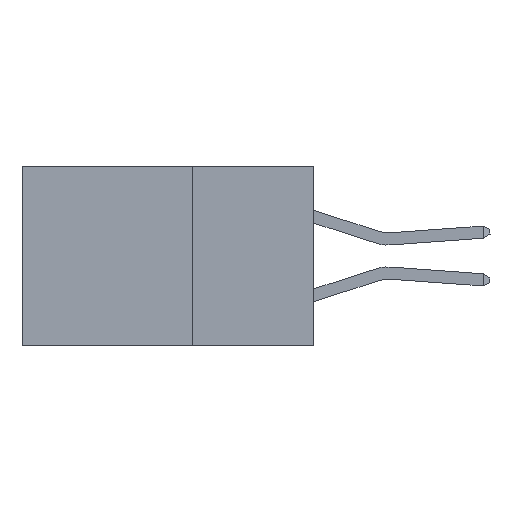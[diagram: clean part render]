
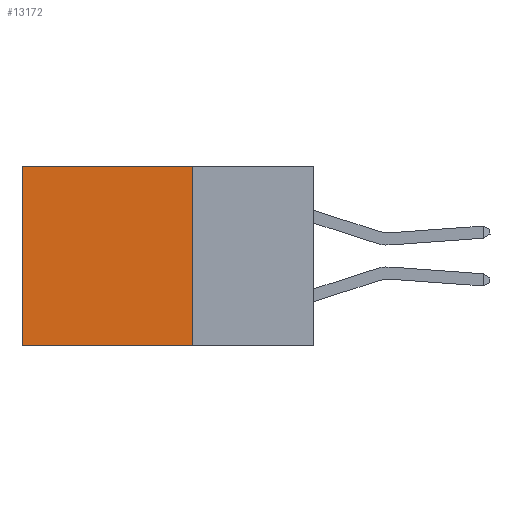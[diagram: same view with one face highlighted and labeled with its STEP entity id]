
A CAD part, left-side view. The second image highlights one B-rep face of the part: STEP entity #13172.
In plain terms, the highlighted planar face has unit normal (-1, 0, 0).
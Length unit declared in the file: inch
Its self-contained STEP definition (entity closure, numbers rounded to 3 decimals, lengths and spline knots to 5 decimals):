
#22 = ORIENTED_EDGE ( 'NONE', *, *, #11337, .F. ) ;
#106 = VECTOR ( 'NONE', #19397, 39.37008 ) ;
#858 = CARTESIAN_POINT ( 'NONE',  ( 0.2875, 0.6, 0. ) ) ;
#1462 = VERTEX_POINT ( 'NONE', #20806 ) ;
#1597 = CARTESIAN_POINT ( 'NONE',  ( 0.2875, 0.25, 0. ) ) ;
#2873 = DIRECTION ( 'NONE',  ( 1., 0., 0. ) ) ;
#3377 = VERTEX_POINT ( 'NONE', #4167 ) ;
#4167 = CARTESIAN_POINT ( 'NONE',  ( 0.2875, 0.25, -0.37 ) ) ;
#4587 = LINE ( 'NONE', #20984, #106 ) ;
#5006 = CARTESIAN_POINT ( 'NONE',  ( 0.2875, 0.6, 0. ) ) ;
#5572 = LINE ( 'NONE', #5006, #8965 ) ;
#5601 = VERTEX_POINT ( 'NONE', #1597 ) ;
#6746 = EDGE_LOOP ( 'NONE', ( #21230, #22, #9424, #15905 ) ) ;
#7415 = CARTESIAN_POINT ( 'NONE',  ( 0.2875, 0.25, 0. ) ) ;
#8239 = CARTESIAN_POINT ( 'NONE',  ( 0.2875, 0.25, -0.37 ) ) ;
#8553 = EDGE_CURVE ( 'NONE', #9463, #1462, #5572, .T. ) ;
#8965 = VECTOR ( 'NONE', #14966, 39.37008 ) ;
#9424 = ORIENTED_EDGE ( 'NONE', *, *, #13683, .F. ) ;
#9463 = VERTEX_POINT ( 'NONE', #858 ) ;
#9910 = DIRECTION ( 'NONE',  ( 0., 1., 0. ) ) ;
#11337 = EDGE_CURVE ( 'NONE', #3377, #1462, #11668, .T. ) ;
#11668 = LINE ( 'NONE', #8239, #19756 ) ;
#12855 = VECTOR ( 'NONE', #15663, 39.37008 ) ;
#13172 = ADVANCED_FACE ( 'NONE', ( #19677 ), #17585, .F. ) ;
#13237 = EDGE_CURVE ( 'NONE', #5601, #9463, #4587, .T. ) ;
#13683 = EDGE_CURVE ( 'NONE', #5601, #3377, #17156, .T. ) ;
#14401 = DIRECTION ( 'NONE',  ( 0., 0., -1. ) ) ;
#14485 = AXIS2_PLACEMENT_3D ( 'NONE', #17520, #2873, #14401 ) ;
#14966 = DIRECTION ( 'NONE',  ( 0., 0., -1. ) ) ;
#15663 = DIRECTION ( 'NONE',  ( 0., 0., -1. ) ) ;
#15905 = ORIENTED_EDGE ( 'NONE', *, *, #13237, .T. ) ;
#17156 = LINE ( 'NONE', #7415, #12855 ) ;
#17520 = CARTESIAN_POINT ( 'NONE',  ( 0.2875, 0.25, 0. ) ) ;
#17585 = PLANE ( 'NONE',  #14485 ) ;
#19397 = DIRECTION ( 'NONE',  ( 0., 1., 0. ) ) ;
#19677 = FACE_OUTER_BOUND ( 'NONE', #6746, .T. ) ;
#19756 = VECTOR ( 'NONE', #9910, 39.37008 ) ;
#20806 = CARTESIAN_POINT ( 'NONE',  ( 0.2875, 0.6, -0.37 ) ) ;
#20984 = CARTESIAN_POINT ( 'NONE',  ( 0.2875, 0.25, 0. ) ) ;
#21230 = ORIENTED_EDGE ( 'NONE', *, *, #8553, .T. ) ;
